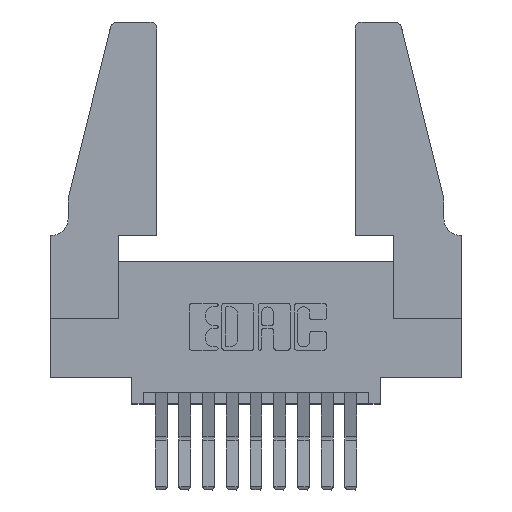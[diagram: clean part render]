
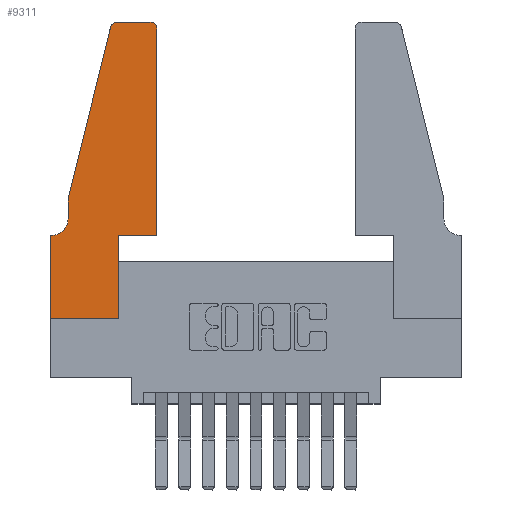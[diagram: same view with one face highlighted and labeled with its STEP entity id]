
A CAD part, top view. The second image highlights one B-rep face of the part: STEP entity #9311.
In plain terms, the highlighted planar face has unit normal (0, 0, 1).
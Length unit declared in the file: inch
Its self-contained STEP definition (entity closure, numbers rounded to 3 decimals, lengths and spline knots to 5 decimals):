
#75 = VECTOR ( 'NONE', #8980, 39.37008 ) ;
#76 = VERTEX_POINT ( 'NONE', #247 ) ;
#98 = CIRCLE ( 'NONE', #1727, 0.07 ) ;
#247 = CARTESIAN_POINT ( 'NONE',  ( 0.0055, 0.35, 0.37 ) ) ;
#369 = DIRECTION ( 'NONE',  ( 1., 0., 0. ) ) ;
#471 = CARTESIAN_POINT ( 'NONE',  ( 0.2605, 1.25, 0.37 ) ) ;
#794 = ORIENTED_EDGE ( 'NONE', *, *, #12519, .T. ) ;
#953 = ORIENTED_EDGE ( 'NONE', *, *, #6620, .T. ) ;
#1006 = EDGE_CURVE ( 'NONE', #10153, #6627, #5721, .T. ) ;
#1359 = CIRCLE ( 'NONE', #6799, 0.03 ) ;
#1380 = VERTEX_POINT ( 'NONE', #4698 ) ;
#1442 = CARTESIAN_POINT ( 'NONE',  ( 0.25487, 1.22718, 0.37 ) ) ;
#1727 = AXIS2_PLACEMENT_3D ( 'NONE', #11864, #2163, #9684 ) ;
#1795 = DIRECTION ( 'NONE',  ( 1., 0., 0. ) ) ;
#1923 = LINE ( 'NONE', #10081, #10109 ) ;
#1930 = CARTESIAN_POINT ( 'NONE',  ( 0.0755, 0.35, 0.37 ) ) ;
#1952 = CARTESIAN_POINT ( 'NONE',  ( 0.0755, 0.5, 0.37 ) ) ;
#2129 = VERTEX_POINT ( 'NONE', #8538 ) ;
#2163 = DIRECTION ( 'NONE',  ( 0., 0., -1. ) ) ;
#2179 = LINE ( 'NONE', #11892, #11914 ) ;
#2291 = LINE ( 'NONE', #5299, #7519 ) ;
#2496 = LINE ( 'NONE', #5193, #7545 ) ;
#2566 = LINE ( 'NONE', #471, #75 ) ;
#2700 = VERTEX_POINT ( 'NONE', #7444 ) ;
#2819 = DIRECTION ( 'NONE',  ( 1., 0., 0. ) ) ;
#2820 = ORIENTED_EDGE ( 'NONE', *, *, #5339, .T. ) ;
#2912 = VERTEX_POINT ( 'NONE', #10831 ) ;
#3277 = CIRCLE ( 'NONE', #12958, 0.03 ) ;
#3323 = DIRECTION ( 'NONE',  ( 0., -1., 0. ) ) ;
#3391 = DIRECTION ( 'NONE',  ( 1., 0., 0. ) ) ;
#3433 = CARTESIAN_POINT ( 'NONE',  ( 0., 0.35, 0.37 ) ) ;
#3474 = LINE ( 'NONE', #1930, #9338 ) ;
#3592 = EDGE_CURVE ( 'NONE', #6627, #2129, #13379, .T. ) ;
#4005 = ORIENTED_EDGE ( 'NONE', *, *, #13410, .T. ) ;
#4559 = AXIS2_PLACEMENT_3D ( 'NONE', #11349, #9161, #2819 ) ;
#4658 = CARTESIAN_POINT ( 'NONE',  ( 0.2865, 0.35, 0.37 ) ) ;
#4698 = CARTESIAN_POINT ( 'NONE',  ( 0.4505, 0.35, 0.37 ) ) ;
#4941 = EDGE_CURVE ( 'NONE', #2700, #6950, #1359, .T. ) ;
#5193 = CARTESIAN_POINT ( 'NONE',  ( 0.4505, 0.35, 0.37 ) ) ;
#5299 = CARTESIAN_POINT ( 'NONE',  ( 0.4505, 0.35, 0.37 ) ) ;
#5339 = EDGE_CURVE ( 'NONE', #6519, #6966, #2179, .T. ) ;
#5721 = LINE ( 'NONE', #10579, #7896 ) ;
#5955 = ORIENTED_EDGE ( 'NONE', *, *, #1006, .T. ) ;
#6295 = DIRECTION ( 'NONE',  ( -1., 0., 0. ) ) ;
#6519 = VERTEX_POINT ( 'NONE', #1952 ) ;
#6620 = EDGE_CURVE ( 'NONE', #10430, #1380, #2496, .T. ) ;
#6627 = VERTEX_POINT ( 'NONE', #7283 ) ;
#6767 = DIRECTION ( 'NONE',  ( 0., 0., 1. ) ) ;
#6799 = AXIS2_PLACEMENT_3D ( 'NONE', #13167, #12017, #3391 ) ;
#6924 = DIRECTION ( 'NONE',  ( 0., 1., 0. ) ) ;
#6950 = VERTEX_POINT ( 'NONE', #8184 ) ;
#6966 = VERTEX_POINT ( 'NONE', #7145 ) ;
#7001 = ORIENTED_EDGE ( 'NONE', *, *, #4941, .T. ) ;
#7129 = FACE_OUTER_BOUND ( 'NONE', #11756, .T. ) ;
#7145 = CARTESIAN_POINT ( 'NONE',  ( 0.0755, 0.42, 0.37 ) ) ;
#7168 = EDGE_CURVE ( 'NONE', #1380, #2700, #2291, .T. ) ;
#7283 = CARTESIAN_POINT ( 'NONE',  ( 0., 0., 0.37 ) ) ;
#7298 = CARTESIAN_POINT ( 'NONE',  ( 0., 0., 0.37 ) ) ;
#7444 = CARTESIAN_POINT ( 'NONE',  ( 0.4505, 1.22, 0.37 ) ) ;
#7492 = EDGE_CURVE ( 'NONE', #76, #10153, #3474, .T. ) ;
#7519 = VECTOR ( 'NONE', #13836, 39.37008 ) ;
#7545 = VECTOR ( 'NONE', #9490, 39.37008 ) ;
#7896 = VECTOR ( 'NONE', #3323, 39.37008 ) ;
#8183 = EDGE_CURVE ( 'NONE', #2912, #9159, #3277, .T. ) ;
#8184 = CARTESIAN_POINT ( 'NONE',  ( 0.4205, 1.25, 0.37 ) ) ;
#8243 = PLANE ( 'NONE',  #4559 ) ;
#8505 = VECTOR ( 'NONE', #13006, 39.37008 ) ;
#8538 = CARTESIAN_POINT ( 'NONE',  ( 0.2865, 0., 0.37 ) ) ;
#8652 = LINE ( 'NONE', #8815, #8505 ) ;
#8815 = CARTESIAN_POINT ( 'NONE',  ( 0.0755, 0.5, 0.37 ) ) ;
#8980 = DIRECTION ( 'NONE',  ( -1., 0., 0. ) ) ;
#9159 = VERTEX_POINT ( 'NONE', #1442 ) ;
#9161 = DIRECTION ( 'NONE',  ( 0., 0., 1. ) ) ;
#9311 = ADVANCED_FACE ( 'NONE', ( #7129 ), #8243, .T. ) ;
#9338 = VECTOR ( 'NONE', #6295, 39.37008 ) ;
#9490 = DIRECTION ( 'NONE',  ( 1., 0., 0. ) ) ;
#9684 = DIRECTION ( 'NONE',  ( -1., 0., 0. ) ) ;
#9852 = ORIENTED_EDGE ( 'NONE', *, *, #3592, .T. ) ;
#10081 = CARTESIAN_POINT ( 'NONE',  ( 0.2865, 0.35, 0.37 ) ) ;
#10109 = VECTOR ( 'NONE', #6924, 39.37008 ) ;
#10153 = VERTEX_POINT ( 'NONE', #3433 ) ;
#10380 = EDGE_CURVE ( 'NONE', #6950, #2912, #2566, .T. ) ;
#10393 = ORIENTED_EDGE ( 'NONE', *, *, #7492, .T. ) ;
#10430 = VERTEX_POINT ( 'NONE', #4658 ) ;
#10579 = CARTESIAN_POINT ( 'NONE',  ( 0., 0., 0.37 ) ) ;
#10831 = CARTESIAN_POINT ( 'NONE',  ( 0.284, 1.25, 0.37 ) ) ;
#11223 = ORIENTED_EDGE ( 'NONE', *, *, #13741, .T. ) ;
#11295 = ORIENTED_EDGE ( 'NONE', *, *, #7168, .T. ) ;
#11349 = CARTESIAN_POINT ( 'NONE',  ( 0., 0.35, 0.37 ) ) ;
#11756 = EDGE_LOOP ( 'NONE', ( #13869, #13906, #794, #2820, #11223, #10393, #5955, #9852, #4005, #953, #11295, #7001 ) ) ;
#11864 = CARTESIAN_POINT ( 'NONE',  ( 0.0055, 0.42, 0.37 ) ) ;
#11892 = CARTESIAN_POINT ( 'NONE',  ( 0.0755, 0.5, 0.37 ) ) ;
#11914 = VECTOR ( 'NONE', #12991, 39.37008 ) ;
#12010 = CARTESIAN_POINT ( 'NONE',  ( 0.284, 1.22, 0.37 ) ) ;
#12017 = DIRECTION ( 'NONE',  ( 0., 0., 1. ) ) ;
#12519 = EDGE_CURVE ( 'NONE', #9159, #6519, #8652, .T. ) ;
#12855 = VECTOR ( 'NONE', #1795, 39.37008 ) ;
#12958 = AXIS2_PLACEMENT_3D ( 'NONE', #12010, #6767, #369 ) ;
#12991 = DIRECTION ( 'NONE',  ( 0., -1., 0. ) ) ;
#13006 = DIRECTION ( 'NONE',  ( -0.239, -0.971, 0. ) ) ;
#13167 = CARTESIAN_POINT ( 'NONE',  ( 0.4205, 1.22, 0.37 ) ) ;
#13379 = LINE ( 'NONE', #7298, #12855 ) ;
#13410 = EDGE_CURVE ( 'NONE', #2129, #10430, #1923, .T. ) ;
#13741 = EDGE_CURVE ( 'NONE', #6966, #76, #98, .T. ) ;
#13836 = DIRECTION ( 'NONE',  ( 0., 1., 0. ) ) ;
#13869 = ORIENTED_EDGE ( 'NONE', *, *, #10380, .T. ) ;
#13906 = ORIENTED_EDGE ( 'NONE', *, *, #8183, .T. ) ;
